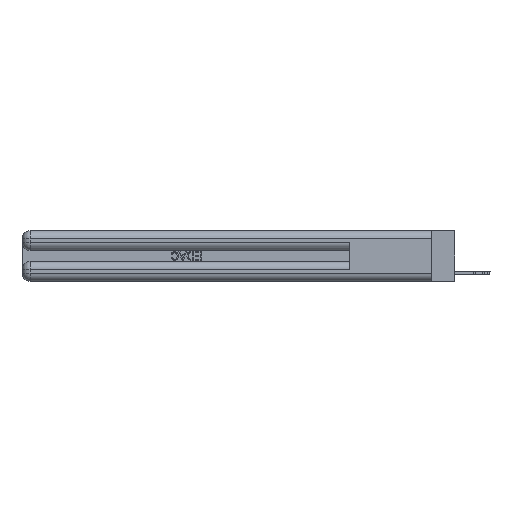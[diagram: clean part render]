
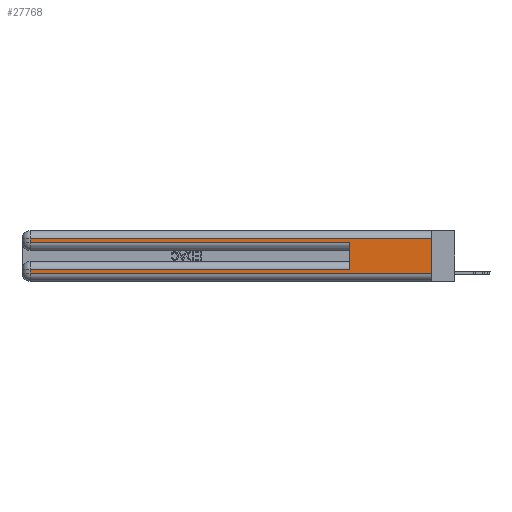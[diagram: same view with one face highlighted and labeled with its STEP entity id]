
A CAD part, left-side view. The second image highlights one B-rep face of the part: STEP entity #27768.
In plain terms, the highlighted planar face has unit normal (-1, 0, 0).
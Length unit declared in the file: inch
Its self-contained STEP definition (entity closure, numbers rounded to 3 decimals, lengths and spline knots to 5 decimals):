
#94 = VERTEX_POINT ( 'NONE', #8079 ) ;
#135 = CARTESIAN_POINT ( 'NONE',  ( 0., 2.94, 0.37 ) ) ;
#378 = ORIENTED_EDGE ( 'NONE', *, *, #1353, .T. ) ;
#950 = DIRECTION ( 'NONE',  ( 0., 1., 0. ) ) ;
#1236 = LINE ( 'NONE', #18329, #14061 ) ;
#1353 = EDGE_CURVE ( 'NONE', #30095, #17534, #6940, .T. ) ;
#1865 = DIRECTION ( 'NONE',  ( 0., -1., 0. ) ) ;
#3119 = ORIENTED_EDGE ( 'NONE', *, *, #6126, .F. ) ;
#3342 = CARTESIAN_POINT ( 'NONE',  ( 0., 0., 0.37 ) ) ;
#3860 = ORIENTED_EDGE ( 'NONE', *, *, #13992, .T. ) ;
#4312 = VECTOR ( 'NONE', #28069, 39.37008 ) ;
#4683 = CARTESIAN_POINT ( 'NONE',  ( 0., 0., 0.31 ) ) ;
#4716 = ORIENTED_EDGE ( 'NONE', *, *, #28349, .F. ) ;
#5085 = VECTOR ( 'NONE', #1865, 39.37008 ) ;
#5087 = VECTOR ( 'NONE', #950, 39.37008 ) ;
#5272 = DIRECTION ( 'NONE',  ( 0., 0., -1. ) ) ;
#5331 = VERTEX_POINT ( 'NONE', #23651 ) ;
#6126 = EDGE_CURVE ( 'NONE', #17805, #27835, #1236, .T. ) ;
#6329 = CARTESIAN_POINT ( 'NONE',  ( 0., 2.94, 0.285 ) ) ;
#6938 = CARTESIAN_POINT ( 'NONE',  ( 0., 0., 0.37 ) ) ;
#6940 = LINE ( 'NONE', #135, #29506 ) ;
#7541 = VECTOR ( 'NONE', #5272, 39.37008 ) ;
#8079 = CARTESIAN_POINT ( 'NONE',  ( 0., 2.94, 0.31 ) ) ;
#8260 = EDGE_LOOP ( 'NONE', ( #4716, #9561, #13595, #3860, #3119, #17897, #378, #23003 ) ) ;
#8841 = FACE_OUTER_BOUND ( 'NONE', #8260, .T. ) ;
#9143 = CARTESIAN_POINT ( 'NONE',  ( 0., 2.94, 0.085 ) ) ;
#9158 = CARTESIAN_POINT ( 'NONE',  ( 0., 0.6, 0.285 ) ) ;
#9561 = ORIENTED_EDGE ( 'NONE', *, *, #19528, .T. ) ;
#10746 = LINE ( 'NONE', #20712, #5087 ) ;
#11548 = PLANE ( 'NONE',  #20149 ) ;
#11928 = DIRECTION ( 'NONE',  ( 0., -1., 0. ) ) ;
#11977 = LINE ( 'NONE', #3342, #7541 ) ;
#13363 = CARTESIAN_POINT ( 'NONE',  ( 0., 2.94, 0.37 ) ) ;
#13595 = ORIENTED_EDGE ( 'NONE', *, *, #25366, .T. ) ;
#13646 = VECTOR ( 'NONE', #11928, 39.37008 ) ;
#13992 = EDGE_CURVE ( 'NONE', #28949, #27835, #18502, .T. ) ;
#14043 = LINE ( 'NONE', #4683, #29036 ) ;
#14061 = VECTOR ( 'NONE', #16273, 39.37008 ) ;
#14243 = DIRECTION ( 'NONE',  ( 0., 0., -1. ) ) ;
#15019 = EDGE_CURVE ( 'NONE', #17805, #30095, #10746, .T. ) ;
#15847 = CARTESIAN_POINT ( 'NONE',  ( 0., 2.94, 0.06 ) ) ;
#16273 = DIRECTION ( 'NONE',  ( 0., 0., 1. ) ) ;
#16615 = DIRECTION ( 'NONE',  ( 0., 0., -1. ) ) ;
#17534 = VERTEX_POINT ( 'NONE', #15847 ) ;
#17805 = VERTEX_POINT ( 'NONE', #23100 ) ;
#17897 = ORIENTED_EDGE ( 'NONE', *, *, #15019, .T. ) ;
#18329 = CARTESIAN_POINT ( 'NONE',  ( 0., 0.6, 0.145 ) ) ;
#18502 = LINE ( 'NONE', #28146, #5085 ) ;
#19041 = CARTESIAN_POINT ( 'NONE',  ( 0., 0., 0.06 ) ) ;
#19398 = DIRECTION ( 'NONE',  ( 0., 1., 0. ) ) ;
#19528 = EDGE_CURVE ( 'NONE', #25565, #94, #14043, .T. ) ;
#20149 = AXIS2_PLACEMENT_3D ( 'NONE', #6938, #30675, #14243 ) ;
#20712 = CARTESIAN_POINT ( 'NONE',  ( 0., 0., 0.085 ) ) ;
#20940 = LINE ( 'NONE', #13363, #4312 ) ;
#21103 = CARTESIAN_POINT ( 'NONE',  ( 0., 0., 0.31 ) ) ;
#23003 = ORIENTED_EDGE ( 'NONE', *, *, #30874, .T. ) ;
#23100 = CARTESIAN_POINT ( 'NONE',  ( 0., 0.6, 0.085 ) ) ;
#23651 = CARTESIAN_POINT ( 'NONE',  ( 0., 0., 0.06 ) ) ;
#25366 = EDGE_CURVE ( 'NONE', #94, #28949, #20940, .T. ) ;
#25565 = VERTEX_POINT ( 'NONE', #21103 ) ;
#27768 = ADVANCED_FACE ( 'NONE', ( #8841 ), #11548, .F. ) ;
#27835 = VERTEX_POINT ( 'NONE', #9158 ) ;
#28069 = DIRECTION ( 'NONE',  ( 0., 0., -1. ) ) ;
#28146 = CARTESIAN_POINT ( 'NONE',  ( 0., 0., 0.285 ) ) ;
#28349 = EDGE_CURVE ( 'NONE', #25565, #5331, #11977, .T. ) ;
#28949 = VERTEX_POINT ( 'NONE', #6329 ) ;
#29036 = VECTOR ( 'NONE', #19398, 39.37008 ) ;
#29506 = VECTOR ( 'NONE', #16615, 39.37008 ) ;
#30095 = VERTEX_POINT ( 'NONE', #9143 ) ;
#30675 = DIRECTION ( 'NONE',  ( 1., 0., 0. ) ) ;
#30737 = LINE ( 'NONE', #19041, #13646 ) ;
#30874 = EDGE_CURVE ( 'NONE', #17534, #5331, #30737, .T. ) ;
